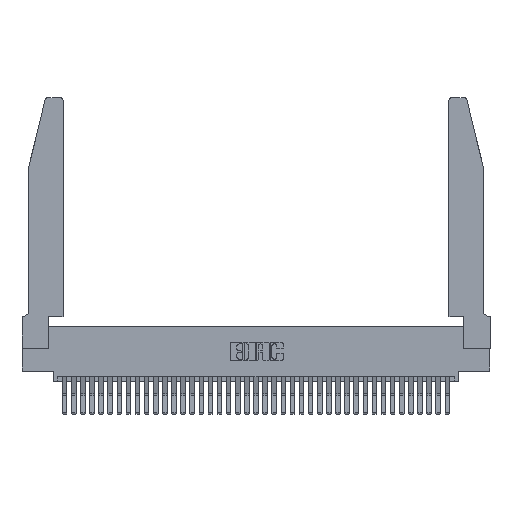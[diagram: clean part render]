
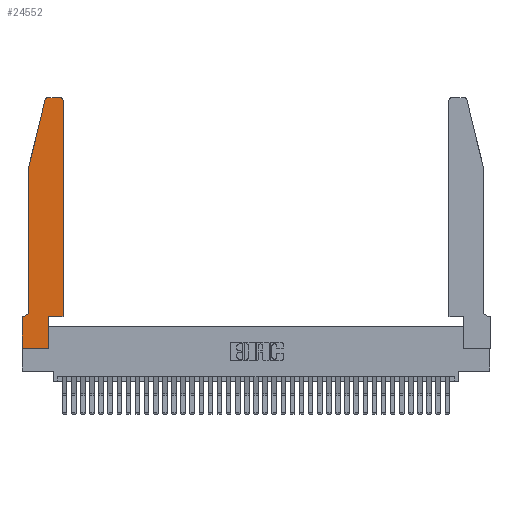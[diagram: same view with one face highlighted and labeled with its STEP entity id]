
A CAD part, top view. The second image highlights one B-rep face of the part: STEP entity #24552.
In plain terms, the highlighted planar face has unit normal (0, 0, 1).
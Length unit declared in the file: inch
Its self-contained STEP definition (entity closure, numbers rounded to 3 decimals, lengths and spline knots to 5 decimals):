
#40 = CARTESIAN_POINT ( 'NONE',  ( 0.284, 2.75, 0.37 ) ) ;
#832 = ORIENTED_EDGE ( 'NONE', *, *, #19200, .T. ) ;
#969 = CARTESIAN_POINT ( 'NONE',  ( 0.2605, 2.75, 0.37 ) ) ;
#1111 = VERTEX_POINT ( 'NONE', #20798 ) ;
#1387 = LINE ( 'NONE', #35100, #31307 ) ;
#1583 = VERTEX_POINT ( 'NONE', #25734 ) ;
#3138 = EDGE_CURVE ( 'NONE', #5400, #29309, #14390, .T. ) ;
#3200 = LINE ( 'NONE', #7397, #26188 ) ;
#3531 = EDGE_CURVE ( 'NONE', #3692, #26222, #9131, .T. ) ;
#3692 = VERTEX_POINT ( 'NONE', #5732 ) ;
#4631 = VECTOR ( 'NONE', #33836, 39.37008 ) ;
#5062 = CARTESIAN_POINT ( 'NONE',  ( 0.4505, 0.35, 0.37 ) ) ;
#5400 = VERTEX_POINT ( 'NONE', #38220 ) ;
#5732 = CARTESIAN_POINT ( 'NONE',  ( 0.4505, 0.35, 0.37 ) ) ;
#5829 = ORIENTED_EDGE ( 'NONE', *, *, #20976, .T. ) ;
#6613 = CARTESIAN_POINT ( 'NONE',  ( 0., 0.35, 0.37 ) ) ;
#6987 = VECTOR ( 'NONE', #35699, 39.37008 ) ;
#7062 = CARTESIAN_POINT ( 'NONE',  ( 0.4505, 2.72, 0.37 ) ) ;
#7184 = AXIS2_PLACEMENT_3D ( 'NONE', #31764, #14168, #34697 ) ;
#7397 = CARTESIAN_POINT ( 'NONE',  ( 0.4505, 0.35, 0.37 ) ) ;
#7669 = ORIENTED_EDGE ( 'NONE', *, *, #20375, .T. ) ;
#8017 = FACE_OUTER_BOUND ( 'NONE', #38257, .T. ) ;
#8411 = ORIENTED_EDGE ( 'NONE', *, *, #3138, .T. ) ;
#8437 = ORIENTED_EDGE ( 'NONE', *, *, #35642, .T. ) ;
#8467 = ORIENTED_EDGE ( 'NONE', *, *, #12474, .T. ) ;
#9131 = LINE ( 'NONE', #5062, #16210 ) ;
#10659 = VECTOR ( 'NONE', #16795, 39.37008 ) ;
#10696 = DIRECTION ( 'NONE',  ( 1., 0., 0. ) ) ;
#10778 = ORIENTED_EDGE ( 'NONE', *, *, #17273, .T. ) ;
#11041 = DIRECTION ( 'NONE',  ( 0., 0., -1. ) ) ;
#12468 = LINE ( 'NONE', #22548, #18563 ) ;
#12474 = EDGE_CURVE ( 'NONE', #16756, #3692, #3200, .T. ) ;
#12589 = EDGE_CURVE ( 'NONE', #26063, #1583, #29344, .T. ) ;
#13696 = LINE ( 'NONE', #969, #4631 ) ;
#14168 = DIRECTION ( 'NONE',  ( 0., 0., 1. ) ) ;
#14173 = ORIENTED_EDGE ( 'NONE', *, *, #3531, .T. ) ;
#14251 = CARTESIAN_POINT ( 'NONE',  ( 0., 0., 0.37 ) ) ;
#14390 = LINE ( 'NONE', #27161, #36867 ) ;
#15006 = CARTESIAN_POINT ( 'NONE',  ( 0., 0.35, 0.37 ) ) ;
#15049 = LINE ( 'NONE', #32746, #6987 ) ;
#15109 = VERTEX_POINT ( 'NONE', #14251 ) ;
#15799 = DIRECTION ( 'NONE',  ( 0., 0., 1. ) ) ;
#16150 = EDGE_CURVE ( 'NONE', #1583, #1111, #33240, .T. ) ;
#16210 = VECTOR ( 'NONE', #31717, 39.37008 ) ;
#16756 = VERTEX_POINT ( 'NONE', #36960 ) ;
#16795 = DIRECTION ( 'NONE',  ( -0.239, -0.971, 0. ) ) ;
#16831 = CARTESIAN_POINT ( 'NONE',  ( 0.0755, 0.42, 0.37 ) ) ;
#17273 = EDGE_CURVE ( 'NONE', #26222, #30144, #29503, .T. ) ;
#17483 = VECTOR ( 'NONE', #23053, 39.37008 ) ;
#17989 = DIRECTION ( 'NONE',  ( 1., 0., 0. ) ) ;
#18466 = EDGE_CURVE ( 'NONE', #15109, #26743, #12468, .T. ) ;
#18563 = VECTOR ( 'NONE', #10696, 39.37008 ) ;
#19200 = EDGE_CURVE ( 'NONE', #21089, #5400, #24911, .T. ) ;
#20375 = EDGE_CURVE ( 'NONE', #26743, #16756, #32133, .T. ) ;
#20798 = CARTESIAN_POINT ( 'NONE',  ( 0.0755, 2., 0.37 ) ) ;
#20976 = EDGE_CURVE ( 'NONE', #30144, #26063, #13696, .T. ) ;
#21089 = VERTEX_POINT ( 'NONE', #16831 ) ;
#21484 = ORIENTED_EDGE ( 'NONE', *, *, #12589, .T. ) ;
#21930 = CARTESIAN_POINT ( 'NONE',  ( 0.4205, 2.75, 0.37 ) ) ;
#22548 = CARTESIAN_POINT ( 'NONE',  ( 0., 0., 0.37 ) ) ;
#23053 = DIRECTION ( 'NONE',  ( 0., 1., 0. ) ) ;
#24552 = ADVANCED_FACE ( 'NONE', ( #8017 ), #26710, .T. ) ;
#24911 = CIRCLE ( 'NONE', #33602, 0.07 ) ;
#25144 = ORIENTED_EDGE ( 'NONE', *, *, #18466, .T. ) ;
#25212 = CARTESIAN_POINT ( 'NONE',  ( 0.2865, 0.35, 0.37 ) ) ;
#25270 = DIRECTION ( 'NONE',  ( 1., 0., 0. ) ) ;
#25734 = CARTESIAN_POINT ( 'NONE',  ( 0.25487, 2.72718, 0.37 ) ) ;
#26063 = VERTEX_POINT ( 'NONE', #40 ) ;
#26188 = VECTOR ( 'NONE', #25270, 39.37008 ) ;
#26222 = VERTEX_POINT ( 'NONE', #7062 ) ;
#26710 = PLANE ( 'NONE',  #32285 ) ;
#26743 = VERTEX_POINT ( 'NONE', #32200 ) ;
#27161 = CARTESIAN_POINT ( 'NONE',  ( 0.0755, 0.35, 0.37 ) ) ;
#28738 = CARTESIAN_POINT ( 'NONE',  ( 0.0055, 0.42, 0.37 ) ) ;
#29040 = EDGE_CURVE ( 'NONE', #29309, #15109, #1387, .T. ) ;
#29309 = VERTEX_POINT ( 'NONE', #6613 ) ;
#29344 = CIRCLE ( 'NONE', #7184, 0.03 ) ;
#29503 = CIRCLE ( 'NONE', #30135, 0.03 ) ;
#30060 = DIRECTION ( 'NONE',  ( -1., 0., 0. ) ) ;
#30135 = AXIS2_PLACEMENT_3D ( 'NONE', #33344, #15799, #36294 ) ;
#30144 = VERTEX_POINT ( 'NONE', #21930 ) ;
#31307 = VECTOR ( 'NONE', #38032, 39.37008 ) ;
#31674 = DIRECTION ( 'NONE',  ( -1., 0., 0. ) ) ;
#31717 = DIRECTION ( 'NONE',  ( 0., 1., 0. ) ) ;
#31764 = CARTESIAN_POINT ( 'NONE',  ( 0.284, 2.72, 0.37 ) ) ;
#32133 = LINE ( 'NONE', #25212, #17483 ) ;
#32200 = CARTESIAN_POINT ( 'NONE',  ( 0.2865, 0., 0.37 ) ) ;
#32285 = AXIS2_PLACEMENT_3D ( 'NONE', #15006, #35498, #17989 ) ;
#32746 = CARTESIAN_POINT ( 'NONE',  ( 0.0755, 2., 0.37 ) ) ;
#33240 = LINE ( 'NONE', #37251, #10659 ) ;
#33344 = CARTESIAN_POINT ( 'NONE',  ( 0.4205, 2.72, 0.37 ) ) ;
#33602 = AXIS2_PLACEMENT_3D ( 'NONE', #28738, #11041, #31674 ) ;
#33836 = DIRECTION ( 'NONE',  ( -1., 0., 0. ) ) ;
#34614 = ORIENTED_EDGE ( 'NONE', *, *, #16150, .T. ) ;
#34697 = DIRECTION ( 'NONE',  ( 1., 0., 0. ) ) ;
#35100 = CARTESIAN_POINT ( 'NONE',  ( 0., 0., 0.37 ) ) ;
#35498 = DIRECTION ( 'NONE',  ( 0., 0., 1. ) ) ;
#35642 = EDGE_CURVE ( 'NONE', #1111, #21089, #15049, .T. ) ;
#35699 = DIRECTION ( 'NONE',  ( 0., -1., 0. ) ) ;
#35964 = ORIENTED_EDGE ( 'NONE', *, *, #29040, .T. ) ;
#36294 = DIRECTION ( 'NONE',  ( 1., 0., 0. ) ) ;
#36867 = VECTOR ( 'NONE', #30060, 39.37008 ) ;
#36960 = CARTESIAN_POINT ( 'NONE',  ( 0.2865, 0.35, 0.37 ) ) ;
#37251 = CARTESIAN_POINT ( 'NONE',  ( 0.0755, 2., 0.37 ) ) ;
#38032 = DIRECTION ( 'NONE',  ( 0., -1., 0. ) ) ;
#38220 = CARTESIAN_POINT ( 'NONE',  ( 0.0055, 0.35, 0.37 ) ) ;
#38257 = EDGE_LOOP ( 'NONE', ( #5829, #21484, #34614, #8437, #832, #8411, #35964, #25144, #7669, #8467, #14173, #10778 ) ) ;
